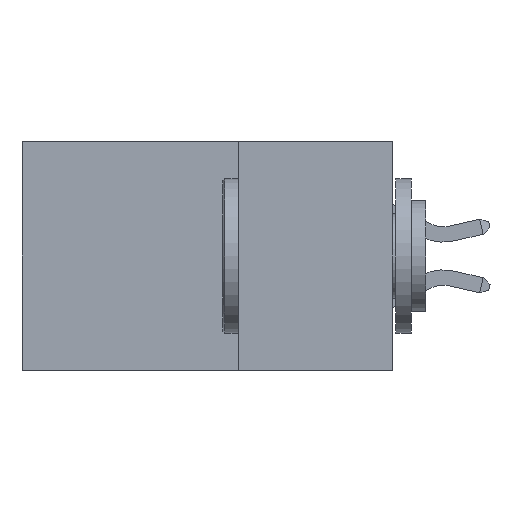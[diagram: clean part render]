
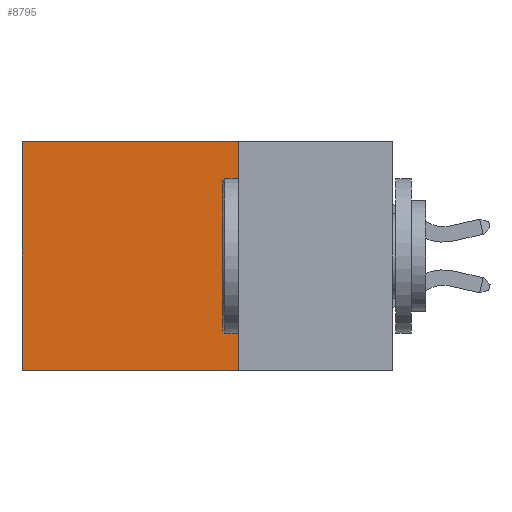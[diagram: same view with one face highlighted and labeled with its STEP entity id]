
A CAD part, left-side view. The second image highlights one B-rep face of the part: STEP entity #8795.
In plain terms, the highlighted planar face has unit normal (-1, 0, 0).
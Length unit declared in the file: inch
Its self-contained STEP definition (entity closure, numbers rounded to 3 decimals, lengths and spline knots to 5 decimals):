
#48 = EDGE_CURVE ( 'NONE', #13118, #7618, #17478, .T. ) ;
#79 = LINE ( 'NONE', #7473, #4653 ) ;
#1344 = DIRECTION ( 'NONE',  ( 0., 1., 0. ) ) ;
#2383 = EDGE_LOOP ( 'NONE', ( #20329, #12655, #10848, #11084 ) ) ;
#3839 = FACE_OUTER_BOUND ( 'NONE', #2383, .T. ) ;
#4653 = VECTOR ( 'NONE', #7547, 39.37008 ) ;
#4990 = CARTESIAN_POINT ( 'NONE',  ( 0.2875, 0.25, 0. ) ) ;
#5192 = EDGE_CURVE ( 'NONE', #19887, #13118, #16392, .T. ) ;
#5655 = LINE ( 'NONE', #11692, #7203 ) ;
#6663 = DIRECTION ( 'NONE',  ( 0., 0., -1. ) ) ;
#7203 = VECTOR ( 'NONE', #13328, 39.37008 ) ;
#7473 = CARTESIAN_POINT ( 'NONE',  ( 0.2875, 0.25, -0.37 ) ) ;
#7547 = DIRECTION ( 'NONE',  ( 0., 1., 0. ) ) ;
#7618 = VERTEX_POINT ( 'NONE', #7625 ) ;
#7625 = CARTESIAN_POINT ( 'NONE',  ( 0.2875, 0.6, -0.37 ) ) ;
#8788 = CARTESIAN_POINT ( 'NONE',  ( 0.2875, 0.25, 0. ) ) ;
#8795 = ADVANCED_FACE ( 'NONE', ( #3839 ), #14468, .F. ) ;
#8821 = AXIS2_PLACEMENT_3D ( 'NONE', #8788, #11671, #19799 ) ;
#9267 = CARTESIAN_POINT ( 'NONE',  ( 0.2875, 0.25, -0.37 ) ) ;
#10848 = ORIENTED_EDGE ( 'NONE', *, *, #20662, .F. ) ;
#11046 = CARTESIAN_POINT ( 'NONE',  ( 0.2875, 0.25, 0. ) ) ;
#11084 = ORIENTED_EDGE ( 'NONE', *, *, #5192, .T. ) ;
#11671 = DIRECTION ( 'NONE',  ( 1., 0., 0. ) ) ;
#11692 = CARTESIAN_POINT ( 'NONE',  ( 0.2875, 0.25, 0. ) ) ;
#12655 = ORIENTED_EDGE ( 'NONE', *, *, #13303, .F. ) ;
#12973 = CARTESIAN_POINT ( 'NONE',  ( 0.2875, 0.6, 0. ) ) ;
#13118 = VERTEX_POINT ( 'NONE', #16278 ) ;
#13303 = EDGE_CURVE ( 'NONE', #15664, #7618, #79, .T. ) ;
#13328 = DIRECTION ( 'NONE',  ( 0., 0., -1. ) ) ;
#14468 = PLANE ( 'NONE',  #8821 ) ;
#15664 = VERTEX_POINT ( 'NONE', #9267 ) ;
#16278 = CARTESIAN_POINT ( 'NONE',  ( 0.2875, 0.6, 0. ) ) ;
#16392 = LINE ( 'NONE', #11046, #20195 ) ;
#17478 = LINE ( 'NONE', #12973, #20248 ) ;
#19799 = DIRECTION ( 'NONE',  ( 0., 0., -1. ) ) ;
#19887 = VERTEX_POINT ( 'NONE', #4990 ) ;
#20195 = VECTOR ( 'NONE', #1344, 39.37008 ) ;
#20248 = VECTOR ( 'NONE', #6663, 39.37008 ) ;
#20329 = ORIENTED_EDGE ( 'NONE', *, *, #48, .T. ) ;
#20662 = EDGE_CURVE ( 'NONE', #19887, #15664, #5655, .T. ) ;
